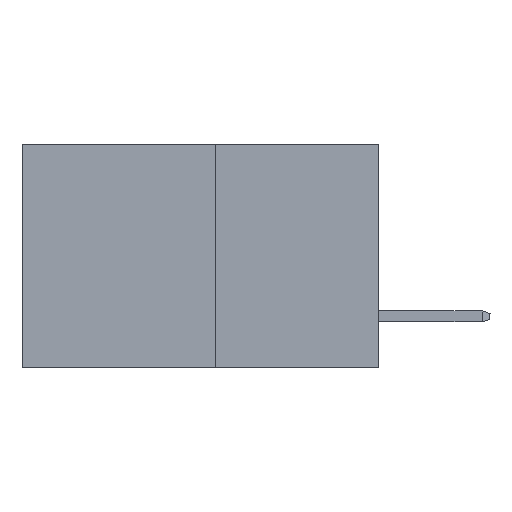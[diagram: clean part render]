
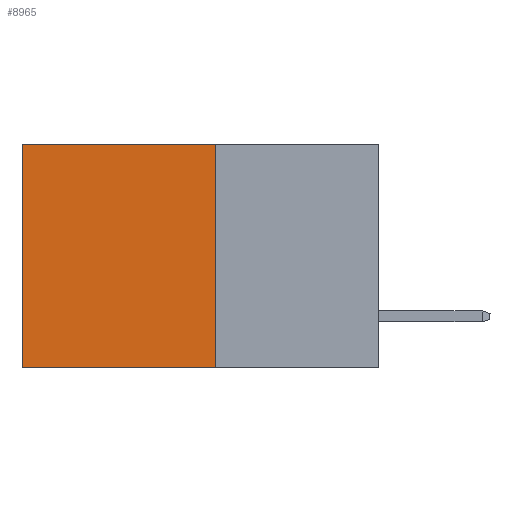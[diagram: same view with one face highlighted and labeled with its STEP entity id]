
A CAD part, left-side view. The second image highlights one B-rep face of the part: STEP entity #8965.
In plain terms, the highlighted planar face has unit normal (-1, 0, 0).
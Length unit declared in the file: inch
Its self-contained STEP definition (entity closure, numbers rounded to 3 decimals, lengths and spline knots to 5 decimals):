
#78 = ORIENTED_EDGE ( 'NONE', *, *, #1432, .F. ) ;
#864 = ORIENTED_EDGE ( 'NONE', *, *, #3326, .F. ) ;
#1082 = ORIENTED_EDGE ( 'NONE', *, *, #1882, .T. ) ;
#1432 = EDGE_CURVE ( 'NONE', #7688, #12793, #11618, .T. ) ;
#1806 = CARTESIAN_POINT ( 'NONE',  ( 0.277, 0.27, -0.37 ) ) ;
#1882 = EDGE_CURVE ( 'NONE', #13498, #2585, #2331, .T. ) ;
#1982 = CARTESIAN_POINT ( 'NONE',  ( 0.277, 0.27, 0. ) ) ;
#2069 = VECTOR ( 'NONE', #7018, 39.37008 ) ;
#2331 = LINE ( 'NONE', #5092, #12612 ) ;
#2416 = VECTOR ( 'NONE', #9855, 39.37008 ) ;
#2585 = VERTEX_POINT ( 'NONE', #8337 ) ;
#3062 = PLANE ( 'NONE',  #5604 ) ;
#3326 = EDGE_CURVE ( 'NONE', #13498, #7688, #10500, .T. ) ;
#4235 = DIRECTION ( 'NONE',  ( 1., 0., 0. ) ) ;
#4833 = EDGE_CURVE ( 'NONE', #2585, #12793, #10760, .T. ) ;
#5092 = CARTESIAN_POINT ( 'NONE',  ( 0.277, 0.27, 0. ) ) ;
#5326 = ORIENTED_EDGE ( 'NONE', *, *, #4833, .T. ) ;
#5604 = AXIS2_PLACEMENT_3D ( 'NONE', #1806, #4235, #11323 ) ;
#6200 = DIRECTION ( 'NONE',  ( 0., 1., 0. ) ) ;
#6524 = FACE_OUTER_BOUND ( 'NONE', #7741, .T. ) ;
#7018 = DIRECTION ( 'NONE',  ( 0., 0., -1. ) ) ;
#7259 = CARTESIAN_POINT ( 'NONE',  ( 0.277, 0.27, -0.37 ) ) ;
#7688 = VERTEX_POINT ( 'NONE', #8068 ) ;
#7741 = EDGE_LOOP ( 'NONE', ( #5326, #78, #864, #1082 ) ) ;
#8068 = CARTESIAN_POINT ( 'NONE',  ( 0.277, 0.27, -0.37 ) ) ;
#8337 = CARTESIAN_POINT ( 'NONE',  ( 0.277, 0.59, 0. ) ) ;
#8965 = ADVANCED_FACE ( 'NONE', ( #6524 ), #3062, .F. ) ;
#9094 = VECTOR ( 'NONE', #11793, 39.37008 ) ;
#9358 = CARTESIAN_POINT ( 'NONE',  ( 0.277, 0.59, -0.37 ) ) ;
#9855 = DIRECTION ( 'NONE',  ( 0., 0., -1. ) ) ;
#10254 = CARTESIAN_POINT ( 'NONE',  ( 0.277, 0.27, -0.37 ) ) ;
#10500 = LINE ( 'NONE', #7259, #2069 ) ;
#10760 = LINE ( 'NONE', #9358, #2416 ) ;
#11323 = DIRECTION ( 'NONE',  ( 0., 0., -1. ) ) ;
#11618 = LINE ( 'NONE', #10254, #9094 ) ;
#11793 = DIRECTION ( 'NONE',  ( 0., 1., 0. ) ) ;
#12612 = VECTOR ( 'NONE', #6200, 39.37008 ) ;
#12793 = VERTEX_POINT ( 'NONE', #13561 ) ;
#13498 = VERTEX_POINT ( 'NONE', #1982 ) ;
#13561 = CARTESIAN_POINT ( 'NONE',  ( 0.277, 0.59, -0.37 ) ) ;
